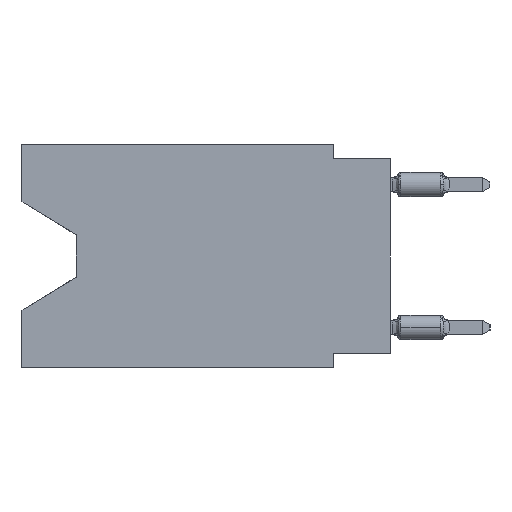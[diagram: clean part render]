
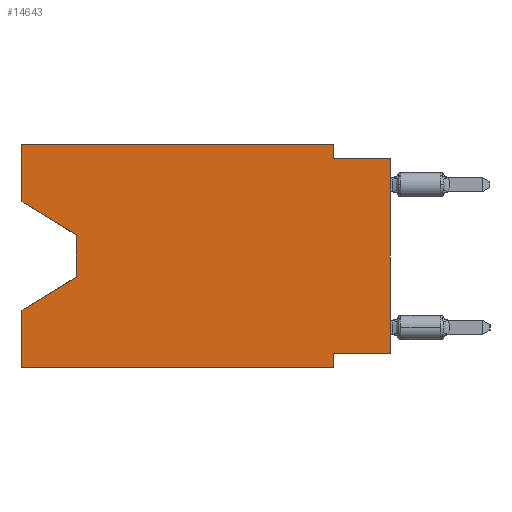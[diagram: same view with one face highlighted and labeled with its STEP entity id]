
A CAD part, left-side view. The second image highlights one B-rep face of the part: STEP entity #14643.
In plain terms, the highlighted planar face has unit normal (-1, 0, 0).
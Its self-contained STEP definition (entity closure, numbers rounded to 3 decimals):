
#21 = CARTESIAN_POINT ( 'NONE',  ( 0., 0., 0. ) ) ;
#295 = VERTEX_POINT ( 'NONE', #16532 ) ;
#619 = PLANE ( 'NONE',  #1579 ) ;
#797 = EDGE_CURVE ( 'NONE', #8891, #24059, #23382, .T. ) ;
#1453 = ORIENTED_EDGE ( 'NONE', *, *, #8393, .F. ) ;
#1579 = AXIS2_PLACEMENT_3D ( 'NONE', #5212, #5504, #16126 ) ;
#1746 = ORIENTED_EDGE ( 'NONE', *, *, #20680, .F. ) ;
#1830 = DIRECTION ( 'NONE',  ( 0., -1., 0. ) ) ;
#2265 = VECTOR ( 'NONE', #8241, 1000. ) ;
#2752 = CARTESIAN_POINT ( 'NONE',  ( 0., 16.383, -2.546 ) ) ;
#3047 = DIRECTION ( 'NONE',  ( 0., 0., -1. ) ) ;
#3359 = VERTEX_POINT ( 'NONE', #15062 ) ;
#3687 = ORIENTED_EDGE ( 'NONE', *, *, #8699, .F. ) ;
#3927 = LINE ( 'NONE', #28197, #2265 ) ;
#4231 = EDGE_LOOP ( 'NONE', ( #19661, #22150, #17252, #1746, #17323, #9366, #11865, #19015, #3687, #18468, #1453, #12658 ) ) ;
#4249 = VECTOR ( 'NONE', #18767, 1000. ) ;
#4423 = VECTOR ( 'NONE', #6647, 1000. ) ;
#4522 = VERTEX_POINT ( 'NONE', #9943 ) ;
#4544 = LINE ( 'NONE', #13721, #23327 ) ;
#5212 = CARTESIAN_POINT ( 'NONE',  ( 0., 16.383, 0. ) ) ;
#5316 = DIRECTION ( 'NONE',  ( 0., 0., -1. ) ) ;
#5504 = DIRECTION ( 'NONE',  ( 1., 0., 0. ) ) ;
#5934 = EDGE_CURVE ( 'NONE', #19791, #9717, #8650, .T. ) ;
#5984 = DIRECTION ( 'NONE',  ( 0., 1., 0. ) ) ;
#6289 = CARTESIAN_POINT ( 'NONE',  ( 0., 13.97, -5.893 ) ) ;
#6411 = CARTESIAN_POINT ( 'NONE',  ( 0., 16.383, -9.906 ) ) ;
#6625 = LINE ( 'NONE', #21, #28178 ) ;
#6647 = DIRECTION ( 'NONE',  ( 0., 0., -1. ) ) ;
#7051 = LINE ( 'NONE', #22979, #20912 ) ;
#8175 = EDGE_CURVE ( 'NONE', #3359, #11825, #22851, .T. ) ;
#8241 = DIRECTION ( 'NONE',  ( 0., -1., 0. ) ) ;
#8393 = EDGE_CURVE ( 'NONE', #16835, #19791, #4544, .T. ) ;
#8650 = LINE ( 'NONE', #22146, #4423 ) ;
#8675 = VECTOR ( 'NONE', #5984, 1000. ) ;
#8699 = EDGE_CURVE ( 'NONE', #9717, #4522, #3927, .T. ) ;
#8846 = DIRECTION ( 'NONE',  ( 0., -1., 0. ) ) ;
#8891 = VERTEX_POINT ( 'NONE', #9244 ) ;
#9107 = VECTOR ( 'NONE', #1830, 1000. ) ;
#9244 = CARTESIAN_POINT ( 'NONE',  ( 0., 0., -9.271 ) ) ;
#9337 = DIRECTION ( 'NONE',  ( 0., -0.855, -0.519 ) ) ;
#9366 = ORIENTED_EDGE ( 'NONE', *, *, #21338, .F. ) ;
#9522 = FACE_OUTER_BOUND ( 'NONE', #4231, .T. ) ;
#9717 = VERTEX_POINT ( 'NONE', #24261 ) ;
#9943 = CARTESIAN_POINT ( 'NONE',  ( 0., 0., -0.635 ) ) ;
#10000 = VECTOR ( 'NONE', #9337, 1000. ) ;
#11655 = LINE ( 'NONE', #15558, #21766 ) ;
#11825 = VERTEX_POINT ( 'NONE', #25308 ) ;
#11865 = ORIENTED_EDGE ( 'NONE', *, *, #797, .F. ) ;
#12658 = ORIENTED_EDGE ( 'NONE', *, *, #26310, .F. ) ;
#12876 = CARTESIAN_POINT ( 'NONE',  ( 0., 16.383, 0. ) ) ;
#13144 = CARTESIAN_POINT ( 'NONE',  ( 0., 2.54, -9.906 ) ) ;
#13465 = CARTESIAN_POINT ( 'NONE',  ( 0., 16.383, 0. ) ) ;
#13721 = CARTESIAN_POINT ( 'NONE',  ( 0., 16.383, 0. ) ) ;
#14037 = CARTESIAN_POINT ( 'NONE',  ( 0., 16.383, 0. ) ) ;
#14182 = VERTEX_POINT ( 'NONE', #13144 ) ;
#14643 = ADVANCED_FACE ( 'NONE', ( #9522 ), #619, .F. ) ;
#14846 = EDGE_CURVE ( 'NONE', #8891, #4522, #6625, .T. ) ;
#15062 = CARTESIAN_POINT ( 'NONE',  ( 0., 16.383, -2.546 ) ) ;
#15329 = LINE ( 'NONE', #13465, #17212 ) ;
#15530 = DIRECTION ( 'NONE',  ( 0., 0., 1. ) ) ;
#15558 = CARTESIAN_POINT ( 'NONE',  ( 0., 13.97, -5.893 ) ) ;
#15834 = CARTESIAN_POINT ( 'NONE',  ( 0., 2.54, 0. ) ) ;
#16097 = CARTESIAN_POINT ( 'NONE',  ( 0., 2.54, -9.906 ) ) ;
#16126 = DIRECTION ( 'NONE',  ( 0., 0., -1. ) ) ;
#16236 = LINE ( 'NONE', #16097, #22889 ) ;
#16494 = CARTESIAN_POINT ( 'NONE',  ( 0., 0., -9.271 ) ) ;
#16532 = CARTESIAN_POINT ( 'NONE',  ( 0., 16.383, -7.36 ) ) ;
#16835 = VERTEX_POINT ( 'NONE', #12876 ) ;
#17018 = CARTESIAN_POINT ( 'NONE',  ( 0., 2.54, -9.271 ) ) ;
#17212 = VECTOR ( 'NONE', #26409, 1000. ) ;
#17252 = ORIENTED_EDGE ( 'NONE', *, *, #26672, .T. ) ;
#17323 = ORIENTED_EDGE ( 'NONE', *, *, #24158, .T. ) ;
#18122 = DIRECTION ( 'NONE',  ( 0., 0.855, -0.519 ) ) ;
#18468 = ORIENTED_EDGE ( 'NONE', *, *, #5934, .F. ) ;
#18767 = DIRECTION ( 'NONE',  ( 0., 0., 1. ) ) ;
#19015 = ORIENTED_EDGE ( 'NONE', *, *, #14846, .T. ) ;
#19459 = LINE ( 'NONE', #6411, #9107 ) ;
#19661 = ORIENTED_EDGE ( 'NONE', *, *, #8175, .T. ) ;
#19791 = VERTEX_POINT ( 'NONE', #15834 ) ;
#20680 = EDGE_CURVE ( 'NONE', #28263, #295, #22662, .T. ) ;
#20912 = VECTOR ( 'NONE', #5316, 1000. ) ;
#21338 = EDGE_CURVE ( 'NONE', #24059, #14182, #16236, .T. ) ;
#21766 = VECTOR ( 'NONE', #18122, 1000. ) ;
#22146 = CARTESIAN_POINT ( 'NONE',  ( 0., 2.54, 0. ) ) ;
#22150 = ORIENTED_EDGE ( 'NONE', *, *, #24926, .T. ) ;
#22662 = LINE ( 'NONE', #14037, #4249 ) ;
#22851 = LINE ( 'NONE', #2752, #10000 ) ;
#22889 = VECTOR ( 'NONE', #3047, 1000. ) ;
#22979 = CARTESIAN_POINT ( 'NONE',  ( 0., 13.97, -4.013 ) ) ;
#23327 = VECTOR ( 'NONE', #8846, 1000. ) ;
#23382 = LINE ( 'NONE', #16494, #8675 ) ;
#24059 = VERTEX_POINT ( 'NONE', #17018 ) ;
#24158 = EDGE_CURVE ( 'NONE', #28263, #14182, #19459, .T. ) ;
#24261 = CARTESIAN_POINT ( 'NONE',  ( 0., 2.54, -0.635 ) ) ;
#24926 = EDGE_CURVE ( 'NONE', #11825, #25273, #7051, .T. ) ;
#25273 = VERTEX_POINT ( 'NONE', #6289 ) ;
#25308 = CARTESIAN_POINT ( 'NONE',  ( 0., 13.97, -4.013 ) ) ;
#26310 = EDGE_CURVE ( 'NONE', #3359, #16835, #15329, .T. ) ;
#26409 = DIRECTION ( 'NONE',  ( 0., 0., 1. ) ) ;
#26672 = EDGE_CURVE ( 'NONE', #25273, #295, #11655, .T. ) ;
#28156 = CARTESIAN_POINT ( 'NONE',  ( 0., 16.383, -9.906 ) ) ;
#28178 = VECTOR ( 'NONE', #15530, 1000. ) ;
#28197 = CARTESIAN_POINT ( 'NONE',  ( 0., 0., -0.635 ) ) ;
#28263 = VERTEX_POINT ( 'NONE', #28156 ) ;
